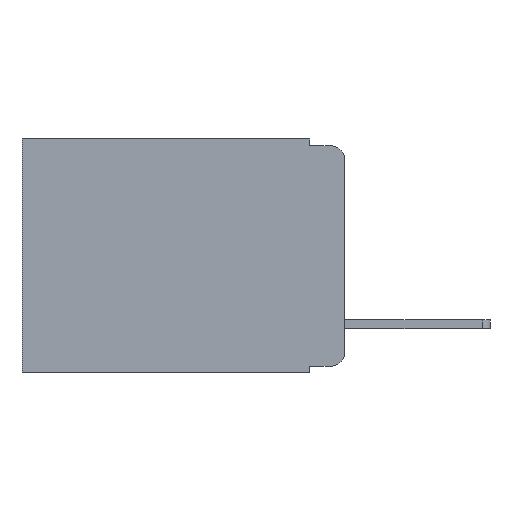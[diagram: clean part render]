
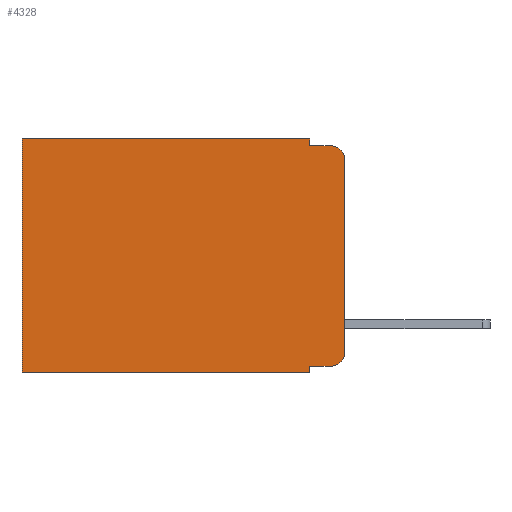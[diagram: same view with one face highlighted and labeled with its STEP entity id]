
A CAD part, left-side view. The second image highlights one B-rep face of the part: STEP entity #4328.
In plain terms, the highlighted planar face has unit normal (-1, 0, 0).
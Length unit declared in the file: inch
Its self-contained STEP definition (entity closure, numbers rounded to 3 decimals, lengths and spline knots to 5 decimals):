
#113 = FACE_OUTER_BOUND ( 'NONE', #4877, .T. ) ;
#131 = CARTESIAN_POINT ( 'NONE',  ( 0.298, 0.02, -0.03 ) ) ;
#152 = VERTEX_POINT ( 'NONE', #5005 ) ;
#477 = CARTESIAN_POINT ( 'NONE',  ( 0.298, 0.051, -0.01 ) ) ;
#878 = LINE ( 'NONE', #6790, #3446 ) ;
#909 = CIRCLE ( 'NONE', #4796, 0.02 ) ;
#980 = DIRECTION ( 'NONE',  ( -1., 0., 0. ) ) ;
#1095 = DIRECTION ( 'NONE',  ( 1., 0., 0. ) ) ;
#1533 = VERTEX_POINT ( 'NONE', #3855 ) ;
#1806 = CIRCLE ( 'NONE', #3264, 0.02 ) ;
#2026 = EDGE_CURVE ( 'NONE', #10104, #9723, #2798, .T. ) ;
#2241 = CARTESIAN_POINT ( 'NONE',  ( 0.298, 0., -0.343 ) ) ;
#2256 = VERTEX_POINT ( 'NONE', #8190 ) ;
#2279 = EDGE_CURVE ( 'NONE', #11626, #10099, #4018, .T. ) ;
#2403 = EDGE_CURVE ( 'NONE', #11626, #152, #12490, .T. ) ;
#2409 = CARTESIAN_POINT ( 'NONE',  ( 0.298, 0., -0.313 ) ) ;
#2470 = VECTOR ( 'NONE', #6150, 39.37008 ) ;
#2502 = EDGE_CURVE ( 'NONE', #152, #9496, #909, .T. ) ;
#2601 = VECTOR ( 'NONE', #10912, 39.37008 ) ;
#2762 = CARTESIAN_POINT ( 'NONE',  ( 0.298, 0.473, 0. ) ) ;
#2798 = LINE ( 'NONE', #2762, #2470 ) ;
#2941 = LINE ( 'NONE', #4520, #3635 ) ;
#2988 = EDGE_CURVE ( 'NONE', #5108, #1533, #1806, .T. ) ;
#3112 = EDGE_CURVE ( 'NONE', #7934, #1533, #2941, .T. ) ;
#3114 = EDGE_CURVE ( 'NONE', #2256, #7934, #7901, .T. ) ;
#3206 = EDGE_CURVE ( 'NONE', #5108, #9496, #878, .T. ) ;
#3264 = AXIS2_PLACEMENT_3D ( 'NONE', #131, #980, #4505 ) ;
#3446 = VECTOR ( 'NONE', #3712, 39.37008 ) ;
#3481 = EDGE_CURVE ( 'NONE', #10099, #9723, #8925, .T. ) ;
#3618 = ORIENTED_EDGE ( 'NONE', *, *, #3206, .F. ) ;
#3635 = VECTOR ( 'NONE', #7714, 39.37008 ) ;
#3644 = ORIENTED_EDGE ( 'NONE', *, *, #2988, .T. ) ;
#3668 = ORIENTED_EDGE ( 'NONE', *, *, #3112, .F. ) ;
#3712 = DIRECTION ( 'NONE',  ( 0., 0., -1. ) ) ;
#3717 = ORIENTED_EDGE ( 'NONE', *, *, #3114, .F. ) ;
#3731 = ORIENTED_EDGE ( 'NONE', *, *, #6208, .T. ) ;
#3843 = ORIENTED_EDGE ( 'NONE', *, *, #2026, .T. ) ;
#3855 = CARTESIAN_POINT ( 'NONE',  ( 0.298, 0.02, -0.01 ) ) ;
#3904 = ORIENTED_EDGE ( 'NONE', *, *, #3481, .F. ) ;
#3917 = ORIENTED_EDGE ( 'NONE', *, *, #2279, .F. ) ;
#3991 = ORIENTED_EDGE ( 'NONE', *, *, #2403, .T. ) ;
#4015 = ORIENTED_EDGE ( 'NONE', *, *, #2502, .T. ) ;
#4018 = LINE ( 'NONE', #7185, #8510 ) ;
#4315 = AXIS2_PLACEMENT_3D ( 'NONE', #9384, #1095, #7244 ) ;
#4328 = ADVANCED_FACE ( 'NONE', ( #113 ), #7278, .F. ) ;
#4505 = DIRECTION ( 'NONE',  ( 0., 0., -1. ) ) ;
#4520 = CARTESIAN_POINT ( 'NONE',  ( 0.298, 0.051, -0.01 ) ) ;
#4796 = AXIS2_PLACEMENT_3D ( 'NONE', #12298, #11124, #6846 ) ;
#4877 = EDGE_LOOP ( 'NONE', ( #3618, #3644, #3668, #3717, #3731, #3843, #3904, #3917, #3991, #4015 ) ) ;
#4906 = CARTESIAN_POINT ( 'NONE',  ( 0.298, 0., 0. ) ) ;
#5005 = CARTESIAN_POINT ( 'NONE',  ( 0.298, 0.02, -0.333 ) ) ;
#5108 = VERTEX_POINT ( 'NONE', #10491 ) ;
#6000 = CARTESIAN_POINT ( 'NONE',  ( 0.298, 0.473, -0.343 ) ) ;
#6150 = DIRECTION ( 'NONE',  ( 0., 0., -1. ) ) ;
#6208 = EDGE_CURVE ( 'NONE', #2256, #10104, #12696, .T. ) ;
#6513 = VECTOR ( 'NONE', #9339, 39.37008 ) ;
#6790 = CARTESIAN_POINT ( 'NONE',  ( 0.298, 0., 0. ) ) ;
#6846 = DIRECTION ( 'NONE',  ( 0., 0., -1. ) ) ;
#6909 = DIRECTION ( 'NONE',  ( 0., 1., 0. ) ) ;
#6934 = CARTESIAN_POINT ( 'NONE',  ( 0.298, 0.051, -0.333 ) ) ;
#7185 = CARTESIAN_POINT ( 'NONE',  ( 0.298, 0.051, 0. ) ) ;
#7244 = DIRECTION ( 'NONE',  ( 0., 0., -1. ) ) ;
#7278 = PLANE ( 'NONE',  #4315 ) ;
#7368 = VECTOR ( 'NONE', #7792, 39.37008 ) ;
#7567 = VECTOR ( 'NONE', #6909, 39.37008 ) ;
#7714 = DIRECTION ( 'NONE',  ( 0., -1., 0. ) ) ;
#7792 = DIRECTION ( 'NONE',  ( 0., -1., 0. ) ) ;
#7901 = LINE ( 'NONE', #10055, #2601 ) ;
#7934 = VERTEX_POINT ( 'NONE', #477 ) ;
#8190 = CARTESIAN_POINT ( 'NONE',  ( 0.298, 0.051, 0. ) ) ;
#8510 = VECTOR ( 'NONE', #9547, 39.37008 ) ;
#8672 = CARTESIAN_POINT ( 'NONE',  ( 0.298, 0.051, -0.343 ) ) ;
#8925 = LINE ( 'NONE', #2241, #6513 ) ;
#9339 = DIRECTION ( 'NONE',  ( 0., 1., 0. ) ) ;
#9384 = CARTESIAN_POINT ( 'NONE',  ( 0.298, 0., 0. ) ) ;
#9496 = VERTEX_POINT ( 'NONE', #2409 ) ;
#9547 = DIRECTION ( 'NONE',  ( 0., 0., -1. ) ) ;
#9723 = VERTEX_POINT ( 'NONE', #6000 ) ;
#10055 = CARTESIAN_POINT ( 'NONE',  ( 0.298, 0.051, 0. ) ) ;
#10099 = VERTEX_POINT ( 'NONE', #8672 ) ;
#10104 = VERTEX_POINT ( 'NONE', #10510 ) ;
#10491 = CARTESIAN_POINT ( 'NONE',  ( 0.298, 0., -0.03 ) ) ;
#10510 = CARTESIAN_POINT ( 'NONE',  ( 0.298, 0.473, 0. ) ) ;
#10607 = CARTESIAN_POINT ( 'NONE',  ( 0.298, 0.051, -0.333 ) ) ;
#10912 = DIRECTION ( 'NONE',  ( 0., 0., -1. ) ) ;
#11124 = DIRECTION ( 'NONE',  ( -1., 0., 0. ) ) ;
#11626 = VERTEX_POINT ( 'NONE', #10607 ) ;
#12298 = CARTESIAN_POINT ( 'NONE',  ( 0.298, 0.02, -0.313 ) ) ;
#12490 = LINE ( 'NONE', #6934, #7368 ) ;
#12696 = LINE ( 'NONE', #4906, #7567 ) ;
